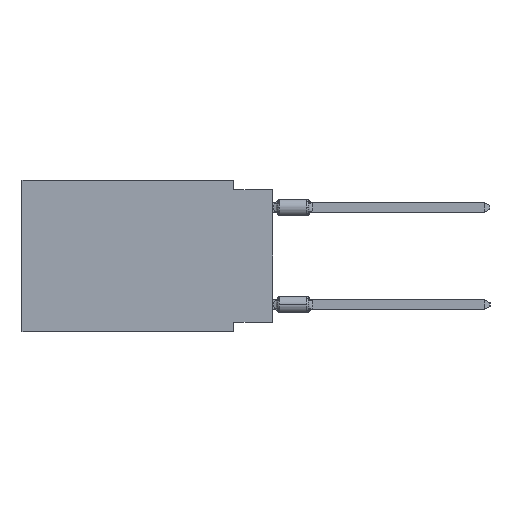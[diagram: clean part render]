
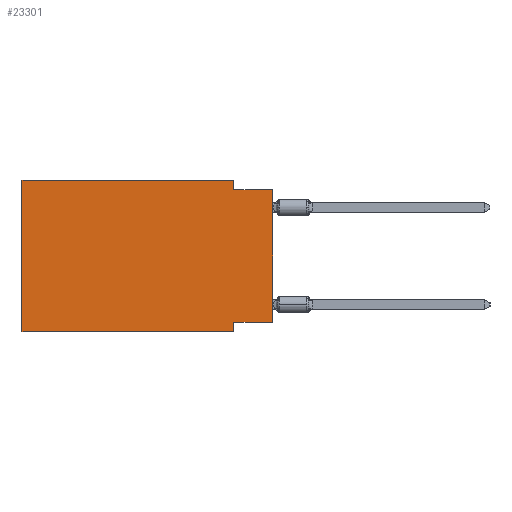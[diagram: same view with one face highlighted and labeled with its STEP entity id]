
A CAD part, left-side view. The second image highlights one B-rep face of the part: STEP entity #23301.
In plain terms, the highlighted planar face has unit normal (-1, 0, 0).
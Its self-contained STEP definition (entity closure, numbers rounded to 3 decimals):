
#1978 = VECTOR ( 'NONE', #50622, 1000. ) ;
#3846 = LINE ( 'NONE', #27072, #14841 ) ;
#4748 = LINE ( 'NONE', #47423, #10441 ) ;
#5646 = VERTEX_POINT ( 'NONE', #18073 ) ;
#6479 = EDGE_LOOP ( 'NONE', ( #59054, #16651, #9878, #27551, #24697, #32567, #47143, #21869 ) ) ;
#7104 = VECTOR ( 'NONE', #43524, 1000. ) ;
#8314 = PLANE ( 'NONE',  #40689 ) ;
#8336 = CARTESIAN_POINT ( 'NONE',  ( 0., 0., -9.271 ) ) ;
#9878 = ORIENTED_EDGE ( 'NONE', *, *, #12504, .F. ) ;
#10315 = CARTESIAN_POINT ( 'NONE',  ( 0., 16.383, -9.906 ) ) ;
#10441 = VECTOR ( 'NONE', #23877, 1000. ) ;
#11734 = CARTESIAN_POINT ( 'NONE',  ( 0., 2.54, 0. ) ) ;
#12504 = EDGE_CURVE ( 'NONE', #61259, #41331, #12863, .T. ) ;
#12863 = LINE ( 'NONE', #23499, #18904 ) ;
#13755 = EDGE_CURVE ( 'NONE', #26251, #31722, #3846, .T. ) ;
#14841 = VECTOR ( 'NONE', #51544, 1000. ) ;
#15176 = EDGE_CURVE ( 'NONE', #5646, #18461, #17974, .T. ) ;
#15650 = LINE ( 'NONE', #10315, #24134 ) ;
#16651 = ORIENTED_EDGE ( 'NONE', *, *, #20844, .F. ) ;
#17118 = EDGE_CURVE ( 'NONE', #26251, #18461, #15650, .T. ) ;
#17143 = DIRECTION ( 'NONE',  ( 0., 1., 0. ) ) ;
#17449 = CARTESIAN_POINT ( 'NONE',  ( 0., 0., -9.271 ) ) ;
#17673 = VERTEX_POINT ( 'NONE', #57174 ) ;
#17974 = LINE ( 'NONE', #37109, #1978 ) ;
#18073 = CARTESIAN_POINT ( 'NONE',  ( 0., 2.54, -9.271 ) ) ;
#18461 = VERTEX_POINT ( 'NONE', #62036 ) ;
#18904 = VECTOR ( 'NONE', #37928, 1000. ) ;
#20844 = EDGE_CURVE ( 'NONE', #41331, #17673, #4748, .T. ) ;
#21869 = ORIENTED_EDGE ( 'NONE', *, *, #57412, .F. ) ;
#23301 = ADVANCED_FACE ( 'NONE', ( #33612 ), #8314, .F. ) ;
#23499 = CARTESIAN_POINT ( 'NONE',  ( 0., 2.54, 0. ) ) ;
#23877 = DIRECTION ( 'NONE',  ( 0., -1., 0. ) ) ;
#24134 = VECTOR ( 'NONE', #29465, 1000. ) ;
#24697 = ORIENTED_EDGE ( 'NONE', *, *, #13755, .F. ) ;
#26251 = VERTEX_POINT ( 'NONE', #61849 ) ;
#27072 = CARTESIAN_POINT ( 'NONE',  ( 0., 16.383, 0. ) ) ;
#27468 = DIRECTION ( 'NONE',  ( 1., 0., 0. ) ) ;
#27551 = ORIENTED_EDGE ( 'NONE', *, *, #44076, .F. ) ;
#29465 = DIRECTION ( 'NONE',  ( 0., -1., 0. ) ) ;
#31722 = VERTEX_POINT ( 'NONE', #42663 ) ;
#32461 = CARTESIAN_POINT ( 'NONE',  ( 0., 16.383, 0. ) ) ;
#32567 = ORIENTED_EDGE ( 'NONE', *, *, #17118, .T. ) ;
#33519 = EDGE_CURVE ( 'NONE', #44204, #17673, #50772, .T. ) ;
#33612 = FACE_OUTER_BOUND ( 'NONE', #6479, .T. ) ;
#35406 = DIRECTION ( 'NONE',  ( 0., 0., 1. ) ) ;
#36340 = CARTESIAN_POINT ( 'NONE',  ( 0., 0., 0. ) ) ;
#37109 = CARTESIAN_POINT ( 'NONE',  ( 0., 2.54, -9.906 ) ) ;
#37928 = DIRECTION ( 'NONE',  ( 0., 0., -1. ) ) ;
#38492 = LINE ( 'NONE', #38799, #7104 ) ;
#38799 = CARTESIAN_POINT ( 'NONE',  ( 0., 16.383, 0. ) ) ;
#40689 = AXIS2_PLACEMENT_3D ( 'NONE', #32461, #27468, #48055 ) ;
#41331 = VERTEX_POINT ( 'NONE', #42780 ) ;
#42041 = VECTOR ( 'NONE', #17143, 1000. ) ;
#42663 = CARTESIAN_POINT ( 'NONE',  ( 0., 16.383, 0. ) ) ;
#42780 = CARTESIAN_POINT ( 'NONE',  ( 0., 2.54, -0.635 ) ) ;
#43524 = DIRECTION ( 'NONE',  ( 0., -1., 0. ) ) ;
#44076 = EDGE_CURVE ( 'NONE', #31722, #61259, #38492, .T. ) ;
#44204 = VERTEX_POINT ( 'NONE', #17449 ) ;
#47143 = ORIENTED_EDGE ( 'NONE', *, *, #15176, .F. ) ;
#47423 = CARTESIAN_POINT ( 'NONE',  ( 0., 0., -0.635 ) ) ;
#48055 = DIRECTION ( 'NONE',  ( 0., 0., -1. ) ) ;
#48587 = VECTOR ( 'NONE', #35406, 1000. ) ;
#50622 = DIRECTION ( 'NONE',  ( 0., 0., -1. ) ) ;
#50772 = LINE ( 'NONE', #36340, #48587 ) ;
#51544 = DIRECTION ( 'NONE',  ( 0., 0., 1. ) ) ;
#55734 = LINE ( 'NONE', #8336, #42041 ) ;
#57174 = CARTESIAN_POINT ( 'NONE',  ( 0., 0., -0.635 ) ) ;
#57412 = EDGE_CURVE ( 'NONE', #44204, #5646, #55734, .T. ) ;
#59054 = ORIENTED_EDGE ( 'NONE', *, *, #33519, .T. ) ;
#61259 = VERTEX_POINT ( 'NONE', #11734 ) ;
#61849 = CARTESIAN_POINT ( 'NONE',  ( 0., 16.383, -9.906 ) ) ;
#62036 = CARTESIAN_POINT ( 'NONE',  ( 0., 2.54, -9.906 ) ) ;
